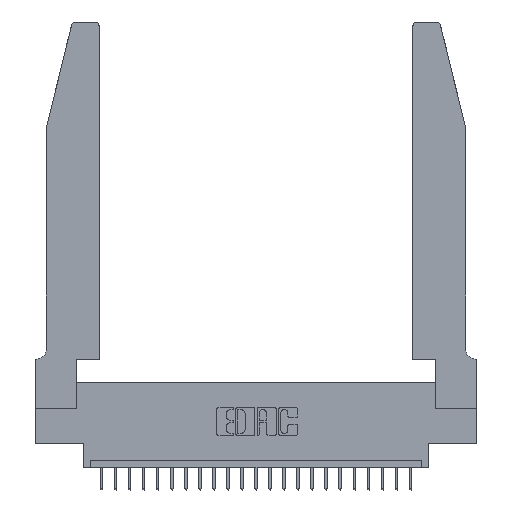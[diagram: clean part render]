
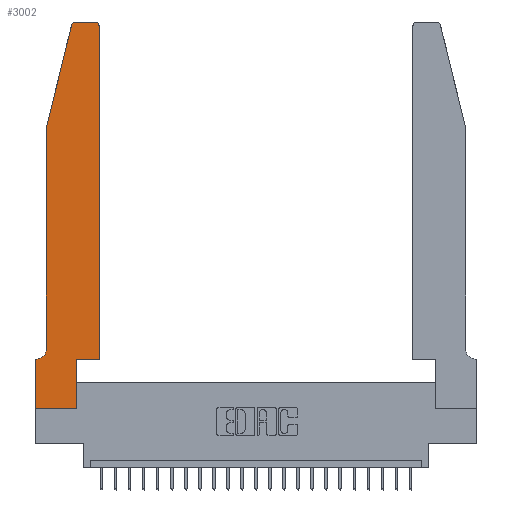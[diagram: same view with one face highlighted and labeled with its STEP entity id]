
A CAD part, top view. The second image highlights one B-rep face of the part: STEP entity #3002.
In plain terms, the highlighted planar face has unit normal (0, 0, 1).
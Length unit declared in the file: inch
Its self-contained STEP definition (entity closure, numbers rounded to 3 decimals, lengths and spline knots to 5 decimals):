
#51 = CARTESIAN_POINT ( 'NONE',  ( 0.0055, 0.35, 0.37 ) ) ;
#484 = DIRECTION ( 'NONE',  ( 0., 0., 1. ) ) ;
#507 = LINE ( 'NONE', #4450, #16677 ) ;
#739 = EDGE_CURVE ( 'NONE', #14714, #20648, #8828, .T. ) ;
#818 = EDGE_CURVE ( 'NONE', #20648, #2577, #13881, .T. ) ;
#1282 = EDGE_LOOP ( 'NONE', ( #23978, #2842, #23789, #9816, #23128, #21336, #23093, #13635, #3954, #6249, #7024, #16599 ) ) ;
#1832 = DIRECTION ( 'NONE',  ( 0., -1., 0. ) ) ;
#1989 = DIRECTION ( 'NONE',  ( 0., 1., 0. ) ) ;
#2074 = DIRECTION ( 'NONE',  ( -1., 0., 0. ) ) ;
#2130 = VECTOR ( 'NONE', #18686, 39.37008 ) ;
#2356 = VERTEX_POINT ( 'NONE', #19550 ) ;
#2412 = CARTESIAN_POINT ( 'NONE',  ( 0.2605, 2.75, 0.37 ) ) ;
#2577 = VERTEX_POINT ( 'NONE', #23457 ) ;
#2668 = DIRECTION ( 'NONE',  ( 1., 0., 0. ) ) ;
#2773 = DIRECTION ( 'NONE',  ( 1., 0., 0. ) ) ;
#2842 = ORIENTED_EDGE ( 'NONE', *, *, #23179, .T. ) ;
#3002 = ADVANCED_FACE ( 'NONE', ( #19842 ), #4551, .T. ) ;
#3032 = CARTESIAN_POINT ( 'NONE',  ( 0., 0.35, 0.37 ) ) ;
#3172 = DIRECTION ( 'NONE',  ( 0., -1., 0. ) ) ;
#3954 = ORIENTED_EDGE ( 'NONE', *, *, #24773, .T. ) ;
#4417 = EDGE_CURVE ( 'NONE', #9881, #19460, #13476, .T. ) ;
#4450 = CARTESIAN_POINT ( 'NONE',  ( 0., 0., 0.37 ) ) ;
#4551 = PLANE ( 'NONE',  #5259 ) ;
#5259 = AXIS2_PLACEMENT_3D ( 'NONE', #3032, #6578, #10446 ) ;
#5671 = CARTESIAN_POINT ( 'NONE',  ( 0.4205, 2.75, 0.37 ) ) ;
#5848 = LINE ( 'NONE', #13329, #16917 ) ;
#6049 = DIRECTION ( 'NONE',  ( -0.239, -0.971, 0. ) ) ;
#6235 = CARTESIAN_POINT ( 'NONE',  ( 0.0055, 0.42, 0.37 ) ) ;
#6249 = ORIENTED_EDGE ( 'NONE', *, *, #24668, .T. ) ;
#6291 = VERTEX_POINT ( 'NONE', #18617 ) ;
#6322 = LINE ( 'NONE', #18250, #23083 ) ;
#6460 = CARTESIAN_POINT ( 'NONE',  ( 0.4505, 0.35, 0.37 ) ) ;
#6578 = DIRECTION ( 'NONE',  ( 0., 0., 1. ) ) ;
#6780 = LINE ( 'NONE', #17396, #13951 ) ;
#7024 = ORIENTED_EDGE ( 'NONE', *, *, #21984, .T. ) ;
#7460 = DIRECTION ( 'NONE',  ( 0., 1., 0. ) ) ;
#7470 = CARTESIAN_POINT ( 'NONE',  ( 0.2865, 0., 0.37 ) ) ;
#8411 = CARTESIAN_POINT ( 'NONE',  ( 0.0755, 2., 0.37 ) ) ;
#8828 = CIRCLE ( 'NONE', #17679, 0.03 ) ;
#9499 = AXIS2_PLACEMENT_3D ( 'NONE', #6235, #12187, #15832 ) ;
#9816 = ORIENTED_EDGE ( 'NONE', *, *, #4417, .T. ) ;
#9881 = VERTEX_POINT ( 'NONE', #8411 ) ;
#9976 = CARTESIAN_POINT ( 'NONE',  ( 0.4205, 2.72, 0.37 ) ) ;
#10446 = DIRECTION ( 'NONE',  ( 1., 0., 0. ) ) ;
#11441 = CIRCLE ( 'NONE', #12763, 0.03 ) ;
#11493 = CIRCLE ( 'NONE', #9499, 0.07 ) ;
#12024 = VECTOR ( 'NONE', #7460, 39.37008 ) ;
#12187 = DIRECTION ( 'NONE',  ( 0., 0., -1. ) ) ;
#12198 = EDGE_CURVE ( 'NONE', #22333, #20030, #507, .T. ) ;
#12242 = CARTESIAN_POINT ( 'NONE',  ( 0.284, 2.72, 0.37 ) ) ;
#12694 = DIRECTION ( 'NONE',  ( 1., 0., 0. ) ) ;
#12763 = AXIS2_PLACEMENT_3D ( 'NONE', #12242, #14147, #2668 ) ;
#13028 = CARTESIAN_POINT ( 'NONE',  ( 0.4505, 2.72, 0.37 ) ) ;
#13329 = CARTESIAN_POINT ( 'NONE',  ( 0., 0., 0.37 ) ) ;
#13476 = LINE ( 'NONE', #20354, #14942 ) ;
#13635 = ORIENTED_EDGE ( 'NONE', *, *, #12198, .T. ) ;
#13881 = LINE ( 'NONE', #2412, #15057 ) ;
#13951 = VECTOR ( 'NONE', #6049, 39.37008 ) ;
#14147 = DIRECTION ( 'NONE',  ( 0., 0., 1. ) ) ;
#14714 = VERTEX_POINT ( 'NONE', #13028 ) ;
#14730 = CARTESIAN_POINT ( 'NONE',  ( 0., 0., 0.37 ) ) ;
#14942 = VECTOR ( 'NONE', #3172, 39.37008 ) ;
#15057 = VECTOR ( 'NONE', #2074, 39.37008 ) ;
#15378 = VERTEX_POINT ( 'NONE', #18354 ) ;
#15832 = DIRECTION ( 'NONE',  ( -1., 0., 0. ) ) ;
#16599 = ORIENTED_EDGE ( 'NONE', *, *, #739, .T. ) ;
#16677 = VECTOR ( 'NONE', #2773, 39.37008 ) ;
#16917 = VECTOR ( 'NONE', #1832, 39.37008 ) ;
#17396 = CARTESIAN_POINT ( 'NONE',  ( 0.0755, 2., 0.37 ) ) ;
#17403 = LINE ( 'NONE', #20543, #2130 ) ;
#17644 = DIRECTION ( 'NONE',  ( 1., 0., 0. ) ) ;
#17679 = AXIS2_PLACEMENT_3D ( 'NONE', #9976, #484, #17644 ) ;
#18250 = CARTESIAN_POINT ( 'NONE',  ( 0.4505, 0.35, 0.37 ) ) ;
#18354 = CARTESIAN_POINT ( 'NONE',  ( 0.25487, 2.72718, 0.37 ) ) ;
#18617 = CARTESIAN_POINT ( 'NONE',  ( 0.4505, 0.35, 0.37 ) ) ;
#18686 = DIRECTION ( 'NONE',  ( -1., 0., 0. ) ) ;
#19460 = VERTEX_POINT ( 'NONE', #23003 ) ;
#19550 = CARTESIAN_POINT ( 'NONE',  ( 0., 0.35, 0.37 ) ) ;
#19842 = FACE_OUTER_BOUND ( 'NONE', #1282, .T. ) ;
#20030 = VERTEX_POINT ( 'NONE', #7470 ) ;
#20070 = LINE ( 'NONE', #24452, #12024 ) ;
#20080 = EDGE_CURVE ( 'NONE', #2356, #22333, #5848, .T. ) ;
#20170 = EDGE_CURVE ( 'NONE', #15378, #9881, #6780, .T. ) ;
#20171 = LINE ( 'NONE', #6460, #20761 ) ;
#20354 = CARTESIAN_POINT ( 'NONE',  ( 0.0755, 2., 0.37 ) ) ;
#20543 = CARTESIAN_POINT ( 'NONE',  ( 0.0755, 0.35, 0.37 ) ) ;
#20648 = VERTEX_POINT ( 'NONE', #5671 ) ;
#20761 = VECTOR ( 'NONE', #1989, 39.37008 ) ;
#21336 = ORIENTED_EDGE ( 'NONE', *, *, #24074, .T. ) ;
#21544 = EDGE_CURVE ( 'NONE', #19460, #22480, #11493, .T. ) ;
#21984 = EDGE_CURVE ( 'NONE', #6291, #14714, #20171, .T. ) ;
#22333 = VERTEX_POINT ( 'NONE', #14730 ) ;
#22480 = VERTEX_POINT ( 'NONE', #51 ) ;
#22927 = VERTEX_POINT ( 'NONE', #24463 ) ;
#23003 = CARTESIAN_POINT ( 'NONE',  ( 0.0755, 0.42, 0.37 ) ) ;
#23083 = VECTOR ( 'NONE', #12694, 39.37008 ) ;
#23093 = ORIENTED_EDGE ( 'NONE', *, *, #20080, .T. ) ;
#23128 = ORIENTED_EDGE ( 'NONE', *, *, #21544, .T. ) ;
#23179 = EDGE_CURVE ( 'NONE', #2577, #15378, #11441, .T. ) ;
#23457 = CARTESIAN_POINT ( 'NONE',  ( 0.284, 2.75, 0.37 ) ) ;
#23789 = ORIENTED_EDGE ( 'NONE', *, *, #20170, .T. ) ;
#23978 = ORIENTED_EDGE ( 'NONE', *, *, #818, .T. ) ;
#24074 = EDGE_CURVE ( 'NONE', #22480, #2356, #17403, .T. ) ;
#24452 = CARTESIAN_POINT ( 'NONE',  ( 0.2865, 0.35, 0.37 ) ) ;
#24463 = CARTESIAN_POINT ( 'NONE',  ( 0.2865, 0.35, 0.37 ) ) ;
#24668 = EDGE_CURVE ( 'NONE', #22927, #6291, #6322, .T. ) ;
#24773 = EDGE_CURVE ( 'NONE', #20030, #22927, #20070, .T. ) ;
